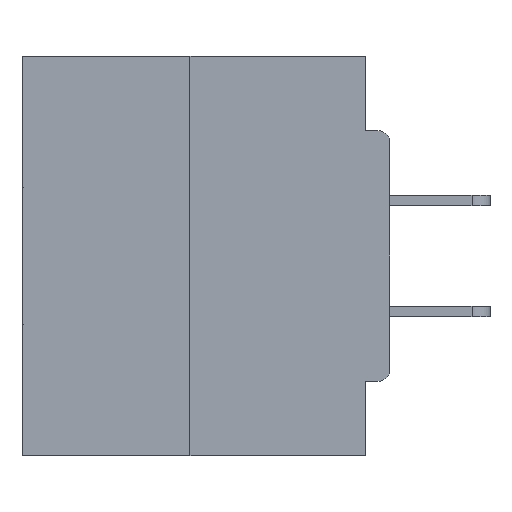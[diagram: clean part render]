
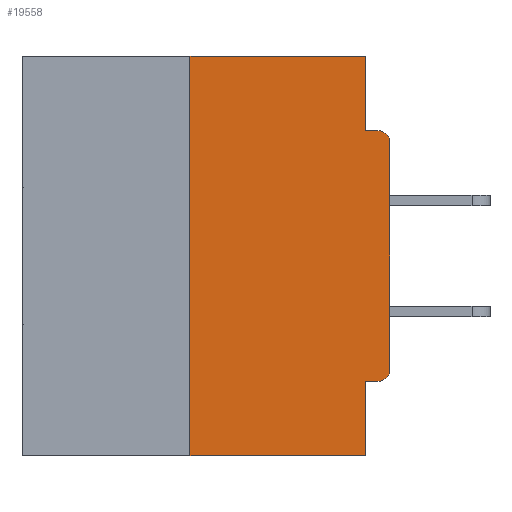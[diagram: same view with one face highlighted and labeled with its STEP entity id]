
A CAD part, left-side view. The second image highlights one B-rep face of the part: STEP entity #19558.
In plain terms, the highlighted planar face has unit normal (-1, 0, 0).
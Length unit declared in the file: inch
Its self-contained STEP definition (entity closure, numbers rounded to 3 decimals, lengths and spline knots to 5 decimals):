
#649 = VERTEX_POINT ( 'NONE', #32562 ) ;
#749 = CARTESIAN_POINT ( 'NONE',  ( 0., 0., -0.4065 ) ) ;
#1079 = LINE ( 'NONE', #30913, #1565 ) ;
#1147 = CARTESIAN_POINT ( 'NONE',  ( 0., 0., 0. ) ) ;
#1565 = VECTOR ( 'NONE', #13491, 39.37008 ) ;
#1844 = LINE ( 'NONE', #10602, #20244 ) ;
#1998 = ORIENTED_EDGE ( 'NONE', *, *, #34751, .T. ) ;
#2599 = ORIENTED_EDGE ( 'NONE', *, *, #33164, .F. ) ;
#2614 = DIRECTION ( 'NONE',  ( -1., 0., 0. ) ) ;
#2690 = CIRCLE ( 'NONE', #5232, 0.015 ) ;
#2798 = CARTESIAN_POINT ( 'NONE',  ( 0., 0.46, 0. ) ) ;
#3175 = EDGE_CURVE ( 'NONE', #4623, #649, #22400, .T. ) ;
#3212 = EDGE_CURVE ( 'NONE', #11321, #25500, #2690, .T. ) ;
#4442 = EDGE_CURVE ( 'NONE', #36204, #25500, #20998, .T. ) ;
#4623 = VERTEX_POINT ( 'NONE', #19350 ) ;
#4625 = DIRECTION ( 'NONE',  ( 0., 0., 1. ) ) ;
#5196 = VERTEX_POINT ( 'NONE', #35367 ) ;
#5232 = AXIS2_PLACEMENT_3D ( 'NONE', #34963, #37663, #26342 ) ;
#5342 = VECTOR ( 'NONE', #8457, 39.37008 ) ;
#5572 = CARTESIAN_POINT ( 'NONE',  ( 0., 0.015, -0.3915 ) ) ;
#5605 = ORIENTED_EDGE ( 'NONE', *, *, #21510, .F. ) ;
#5901 = DIRECTION ( 'NONE',  ( 0., 0., -1. ) ) ;
#6257 = VECTOR ( 'NONE', #4625, 39.37008 ) ;
#6508 = CARTESIAN_POINT ( 'NONE',  ( 0., 0., -0.1085 ) ) ;
#6590 = EDGE_CURVE ( 'NONE', #30105, #23918, #1079, .T. ) ;
#6757 = VERTEX_POINT ( 'NONE', #14611 ) ;
#8191 = CARTESIAN_POINT ( 'NONE',  ( 0., 0.031, -0.5 ) ) ;
#8457 = DIRECTION ( 'NONE',  ( 0., 0., -1. ) ) ;
#8525 = LINE ( 'NONE', #12499, #23174 ) ;
#10078 = DIRECTION ( 'NONE',  ( 0., -1., 0. ) ) ;
#10602 = CARTESIAN_POINT ( 'NONE',  ( 0., 0.46, -0.5 ) ) ;
#11321 = VERTEX_POINT ( 'NONE', #6508 ) ;
#12499 = CARTESIAN_POINT ( 'NONE',  ( 0., 0.25, 0. ) ) ;
#12765 = EDGE_CURVE ( 'NONE', #6757, #30105, #8525, .T. ) ;
#13147 = LINE ( 'NONE', #1147, #6257 ) ;
#13163 = LINE ( 'NONE', #8191, #5342 ) ;
#13491 = DIRECTION ( 'NONE',  ( 0., -1., 0. ) ) ;
#14229 = CARTESIAN_POINT ( 'NONE',  ( 0., 0.031, 0. ) ) ;
#14611 = CARTESIAN_POINT ( 'NONE',  ( 0., 0.25, -0.5 ) ) ;
#15663 = CARTESIAN_POINT ( 'NONE',  ( 0., 0.25, 0. ) ) ;
#15999 = ORIENTED_EDGE ( 'NONE', *, *, #20084, .T. ) ;
#16015 = DIRECTION ( 'NONE',  ( 0., 1., 0. ) ) ;
#17501 = ORIENTED_EDGE ( 'NONE', *, *, #3175, .T. ) ;
#18787 = CARTESIAN_POINT ( 'NONE',  ( 0., 0., -0.0935 ) ) ;
#19350 = CARTESIAN_POINT ( 'NONE',  ( 0., 0.015, -0.4065 ) ) ;
#19558 = ADVANCED_FACE ( 'NONE', ( #28548 ), #20003, .F. ) ;
#19915 = VECTOR ( 'NONE', #16015, 39.37008 ) ;
#20003 = PLANE ( 'NONE',  #27248 ) ;
#20084 = EDGE_CURVE ( 'NONE', #6757, #36048, #1844, .T. ) ;
#20117 = DIRECTION ( 'NONE',  ( 0., 0., -1. ) ) ;
#20244 = VECTOR ( 'NONE', #36918, 39.37008 ) ;
#20374 = DIRECTION ( 'NONE',  ( 1., 0., 0. ) ) ;
#20998 = LINE ( 'NONE', #18787, #25107 ) ;
#21299 = CARTESIAN_POINT ( 'NONE',  ( 0., 0.031, 0. ) ) ;
#21471 = AXIS2_PLACEMENT_3D ( 'NONE', #5572, #2614, #26089 ) ;
#21510 = EDGE_CURVE ( 'NONE', #4623, #5196, #30039, .T. ) ;
#21782 = DIRECTION ( 'NONE',  ( 0., 0., 1. ) ) ;
#22400 = CIRCLE ( 'NONE', #21471, 0.015 ) ;
#22578 = ORIENTED_EDGE ( 'NONE', *, *, #3212, .T. ) ;
#22992 = EDGE_CURVE ( 'NONE', #23918, #36204, #31738, .T. ) ;
#23174 = VECTOR ( 'NONE', #21782, 39.37008 ) ;
#23918 = VERTEX_POINT ( 'NONE', #21299 ) ;
#25107 = VECTOR ( 'NONE', #10078, 39.37008 ) ;
#25500 = VERTEX_POINT ( 'NONE', #34538 ) ;
#26089 = DIRECTION ( 'NONE',  ( 0., 0., -1. ) ) ;
#26342 = DIRECTION ( 'NONE',  ( 0., 0., -1. ) ) ;
#27248 = AXIS2_PLACEMENT_3D ( 'NONE', #2798, #20374, #5901 ) ;
#28548 = FACE_OUTER_BOUND ( 'NONE', #29653, .T. ) ;
#28987 = VECTOR ( 'NONE', #20117, 39.37008 ) ;
#29653 = EDGE_LOOP ( 'NONE', ( #36519, #31780, #15999, #2599, #5605, #17501, #1998, #22578, #33559, #29883 ) ) ;
#29883 = ORIENTED_EDGE ( 'NONE', *, *, #22992, .F. ) ;
#30039 = LINE ( 'NONE', #749, #19915 ) ;
#30105 = VERTEX_POINT ( 'NONE', #15663 ) ;
#30569 = CARTESIAN_POINT ( 'NONE',  ( 0., 0.031, -0.0935 ) ) ;
#30913 = CARTESIAN_POINT ( 'NONE',  ( 0., 0.46, 0. ) ) ;
#31349 = CARTESIAN_POINT ( 'NONE',  ( 0., 0.031, -0.5 ) ) ;
#31738 = LINE ( 'NONE', #14229, #28987 ) ;
#31780 = ORIENTED_EDGE ( 'NONE', *, *, #12765, .F. ) ;
#32562 = CARTESIAN_POINT ( 'NONE',  ( 0., 0., -0.3915 ) ) ;
#33164 = EDGE_CURVE ( 'NONE', #5196, #36048, #13163, .T. ) ;
#33559 = ORIENTED_EDGE ( 'NONE', *, *, #4442, .F. ) ;
#34538 = CARTESIAN_POINT ( 'NONE',  ( 0., 0.015, -0.0935 ) ) ;
#34751 = EDGE_CURVE ( 'NONE', #649, #11321, #13147, .T. ) ;
#34963 = CARTESIAN_POINT ( 'NONE',  ( 0., 0.015, -0.1085 ) ) ;
#35367 = CARTESIAN_POINT ( 'NONE',  ( 0., 0.031, -0.4065 ) ) ;
#36048 = VERTEX_POINT ( 'NONE', #31349 ) ;
#36204 = VERTEX_POINT ( 'NONE', #30569 ) ;
#36519 = ORIENTED_EDGE ( 'NONE', *, *, #6590, .F. ) ;
#36918 = DIRECTION ( 'NONE',  ( 0., -1., 0. ) ) ;
#37663 = DIRECTION ( 'NONE',  ( -1., 0., 0. ) ) ;
